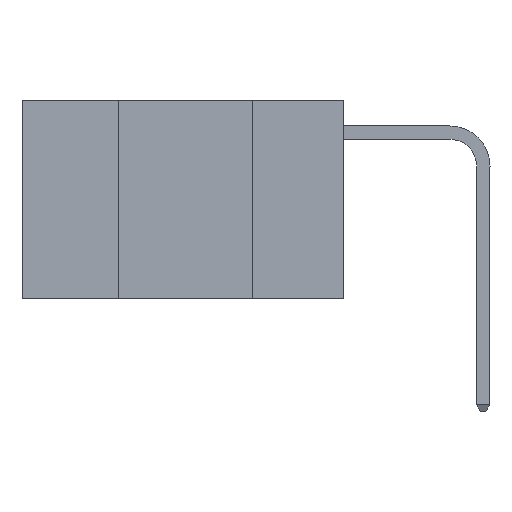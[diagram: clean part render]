
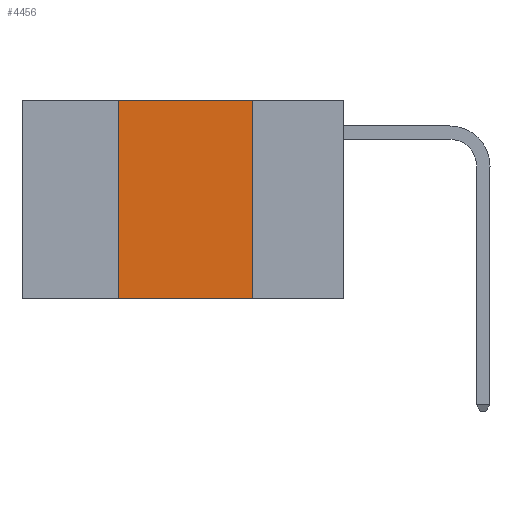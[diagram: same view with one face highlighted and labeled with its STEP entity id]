
A CAD part, left-side view. The second image highlights one B-rep face of the part: STEP entity #4456.
In plain terms, the highlighted planar face has unit normal (-1, 0, 0).
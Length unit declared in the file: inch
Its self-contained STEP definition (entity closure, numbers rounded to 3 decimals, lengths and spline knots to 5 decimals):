
#255 = EDGE_LOOP ( 'NONE', ( #5637, #9661, #16344, #19977 ) ) ;
#711 = EDGE_CURVE ( 'NONE', #19783, #9582, #11784, .T. ) ;
#886 = DIRECTION ( 'NONE',  ( 0., 0., -1. ) ) ;
#963 = CARTESIAN_POINT ( 'NONE',  ( 0., 0.6, -0.37 ) ) ;
#1756 = PLANE ( 'NONE',  #18452 ) ;
#2113 = LINE ( 'NONE', #963, #11426 ) ;
#2558 = CARTESIAN_POINT ( 'NONE',  ( 0., 0.17, 0. ) ) ;
#3008 = VECTOR ( 'NONE', #886, 39.37008 ) ;
#3414 = DIRECTION ( 'NONE',  ( 0., 0., -1. ) ) ;
#4456 = ADVANCED_FACE ( 'NONE', ( #6892 ), #1756, .F. ) ;
#5027 = CARTESIAN_POINT ( 'NONE',  ( 0., 0.42, 0. ) ) ;
#5637 = ORIENTED_EDGE ( 'NONE', *, *, #20278, .F. ) ;
#5878 = VECTOR ( 'NONE', #17287, 39.37008 ) ;
#6411 = LINE ( 'NONE', #15748, #5878 ) ;
#6714 = VERTEX_POINT ( 'NONE', #15347 ) ;
#6892 = FACE_OUTER_BOUND ( 'NONE', #255, .T. ) ;
#7392 = EDGE_CURVE ( 'NONE', #19783, #10792, #2113, .T. ) ;
#9582 = VERTEX_POINT ( 'NONE', #5027 ) ;
#9661 = ORIENTED_EDGE ( 'NONE', *, *, #19050, .F. ) ;
#10792 = VERTEX_POINT ( 'NONE', #16673 ) ;
#10925 = DIRECTION ( 'NONE',  ( 0., 0., 1. ) ) ;
#10950 = CARTESIAN_POINT ( 'NONE',  ( 0., 0.42, 0. ) ) ;
#11426 = VECTOR ( 'NONE', #14047, 39.37008 ) ;
#11643 = CARTESIAN_POINT ( 'NONE',  ( 0., 0.6, 0. ) ) ;
#11784 = LINE ( 'NONE', #10950, #15474 ) ;
#13254 = DIRECTION ( 'NONE',  ( 1., 0., 0. ) ) ;
#14047 = DIRECTION ( 'NONE',  ( 0., -1., 0. ) ) ;
#15347 = CARTESIAN_POINT ( 'NONE',  ( 0., 0.17, 0. ) ) ;
#15474 = VECTOR ( 'NONE', #10925, 39.37008 ) ;
#15748 = CARTESIAN_POINT ( 'NONE',  ( 0., 0.6, 0. ) ) ;
#15963 = LINE ( 'NONE', #2558, #3008 ) ;
#16344 = ORIENTED_EDGE ( 'NONE', *, *, #711, .F. ) ;
#16673 = CARTESIAN_POINT ( 'NONE',  ( 0., 0.17, -0.37 ) ) ;
#17287 = DIRECTION ( 'NONE',  ( 0., -1., 0. ) ) ;
#18452 = AXIS2_PLACEMENT_3D ( 'NONE', #11643, #13254, #3414 ) ;
#19050 = EDGE_CURVE ( 'NONE', #9582, #6714, #6411, .T. ) ;
#19783 = VERTEX_POINT ( 'NONE', #20279 ) ;
#19977 = ORIENTED_EDGE ( 'NONE', *, *, #7392, .T. ) ;
#20278 = EDGE_CURVE ( 'NONE', #6714, #10792, #15963, .T. ) ;
#20279 = CARTESIAN_POINT ( 'NONE',  ( 0., 0.42, -0.37 ) ) ;
